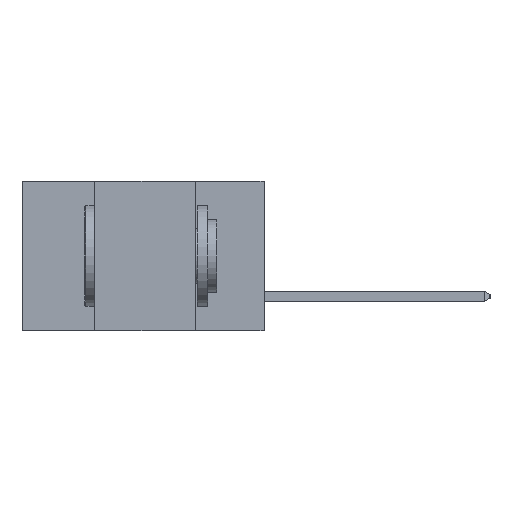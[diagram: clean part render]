
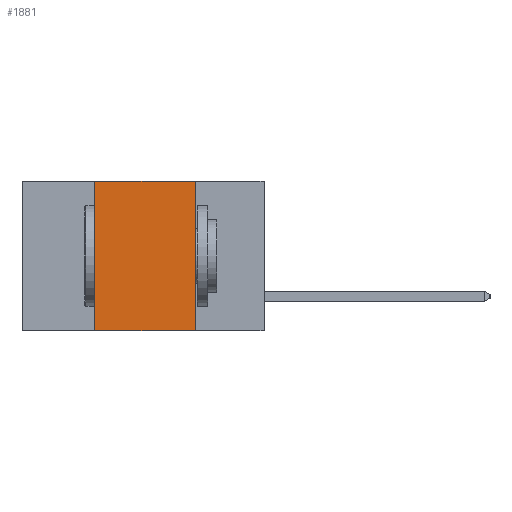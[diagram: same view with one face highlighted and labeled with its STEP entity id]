
A CAD part, left-side view. The second image highlights one B-rep face of the part: STEP entity #1881.
In plain terms, the highlighted planar face has unit normal (-1, 0, 0).
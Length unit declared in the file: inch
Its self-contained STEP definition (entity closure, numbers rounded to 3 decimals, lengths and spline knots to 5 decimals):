
#218 = LINE ( 'NONE', #8481, #10639 ) ;
#254 = CARTESIAN_POINT ( 'NONE',  ( 0., 0.6, 0. ) ) ;
#392 = VECTOR ( 'NONE', #527, 39.37008 ) ;
#527 = DIRECTION ( 'NONE',  ( 0., 0., -1. ) ) ;
#1787 = EDGE_CURVE ( 'NONE', #5852, #16415, #218, .T. ) ;
#1881 = ADVANCED_FACE ( 'NONE', ( #12876 ), #7233, .F. ) ;
#1901 = VERTEX_POINT ( 'NONE', #14047 ) ;
#2171 = ORIENTED_EDGE ( 'NONE', *, *, #9150, .F. ) ;
#2255 = CARTESIAN_POINT ( 'NONE',  ( 0., 0.6, 0. ) ) ;
#4059 = LINE ( 'NONE', #12670, #392 ) ;
#4106 = LINE ( 'NONE', #16226, #10863 ) ;
#4169 = DIRECTION ( 'NONE',  ( 0., 0., 1. ) ) ;
#5852 = VERTEX_POINT ( 'NONE', #15253 ) ;
#6294 = ORIENTED_EDGE ( 'NONE', *, *, #1787, .T. ) ;
#7161 = DIRECTION ( 'NONE',  ( 0., 0., -1. ) ) ;
#7233 = PLANE ( 'NONE',  #16609 ) ;
#8481 = CARTESIAN_POINT ( 'NONE',  ( 0., 0.6, -0.37 ) ) ;
#8500 = VERTEX_POINT ( 'NONE', #14989 ) ;
#9150 = EDGE_CURVE ( 'NONE', #5852, #1901, #4106, .T. ) ;
#10639 = VECTOR ( 'NONE', #13297, 39.37008 ) ;
#10863 = VECTOR ( 'NONE', #4169, 39.37008 ) ;
#11123 = DIRECTION ( 'NONE',  ( 0., -1., 0. ) ) ;
#11730 = VECTOR ( 'NONE', #11123, 39.37008 ) ;
#11791 = EDGE_CURVE ( 'NONE', #1901, #8500, #16046, .T. ) ;
#12670 = CARTESIAN_POINT ( 'NONE',  ( 0., 0.17, -0.37 ) ) ;
#12876 = FACE_OUTER_BOUND ( 'NONE', #12943, .T. ) ;
#12943 = EDGE_LOOP ( 'NONE', ( #15631, #16036, #2171, #6294 ) ) ;
#13297 = DIRECTION ( 'NONE',  ( 0., -1., 0. ) ) ;
#13491 = DIRECTION ( 'NONE',  ( 1., 0., 0. ) ) ;
#14047 = CARTESIAN_POINT ( 'NONE',  ( 0., 0.42, 0. ) ) ;
#14443 = EDGE_CURVE ( 'NONE', #8500, #16415, #4059, .T. ) ;
#14989 = CARTESIAN_POINT ( 'NONE',  ( 0., 0.17, 0. ) ) ;
#15253 = CARTESIAN_POINT ( 'NONE',  ( 0., 0.42, -0.37 ) ) ;
#15613 = CARTESIAN_POINT ( 'NONE',  ( 0., 0.17, -0.37 ) ) ;
#15631 = ORIENTED_EDGE ( 'NONE', *, *, #14443, .F. ) ;
#16036 = ORIENTED_EDGE ( 'NONE', *, *, #11791, .F. ) ;
#16046 = LINE ( 'NONE', #254, #11730 ) ;
#16226 = CARTESIAN_POINT ( 'NONE',  ( 0., 0.42, -0.37 ) ) ;
#16415 = VERTEX_POINT ( 'NONE', #15613 ) ;
#16609 = AXIS2_PLACEMENT_3D ( 'NONE', #2255, #13491, #7161 ) ;
